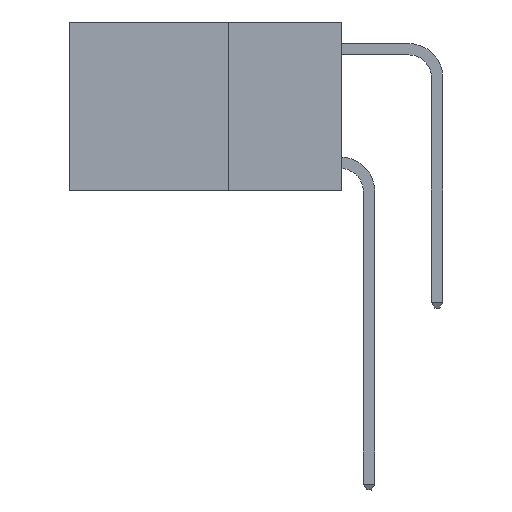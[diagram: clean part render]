
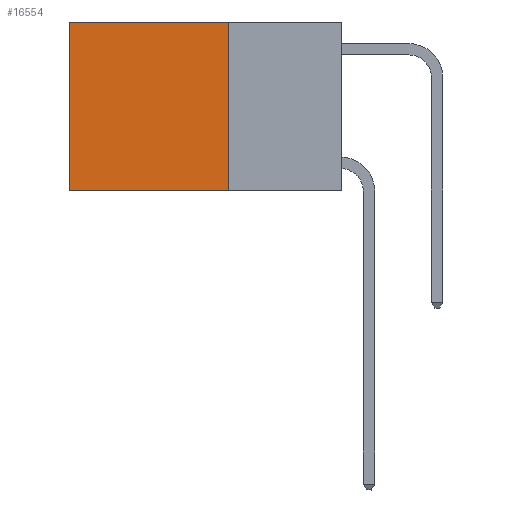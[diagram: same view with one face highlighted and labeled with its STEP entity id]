
A CAD part, left-side view. The second image highlights one B-rep face of the part: STEP entity #16554.
In plain terms, the highlighted planar face has unit normal (-1, 0, 0).
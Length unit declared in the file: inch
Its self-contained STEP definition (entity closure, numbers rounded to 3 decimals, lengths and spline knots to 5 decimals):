
#1660 = DIRECTION ( 'NONE',  ( 0., 1., 0. ) ) ;
#2607 = VECTOR ( 'NONE', #20338, 39.37008 ) ;
#3038 = VERTEX_POINT ( 'NONE', #21489 ) ;
#4496 = EDGE_CURVE ( 'NONE', #20024, #8910, #19858, .T. ) ;
#4910 = LINE ( 'NONE', #21414, #20687 ) ;
#5083 = EDGE_CURVE ( 'NONE', #3038, #20024, #23173, .T. ) ;
#5588 = CARTESIAN_POINT ( 'NONE',  ( 0.2625, 0.25, 0. ) ) ;
#6505 = CARTESIAN_POINT ( 'NONE',  ( 0.2625, 0.25, 0. ) ) ;
#6609 = ORIENTED_EDGE ( 'NONE', *, *, #5083, .T. ) ;
#6705 = AXIS2_PLACEMENT_3D ( 'NONE', #19787, #7940, #21731 ) ;
#7940 = DIRECTION ( 'NONE',  ( 1., 0., 0. ) ) ;
#8168 = EDGE_CURVE ( 'NONE', #3038, #17429, #18433, .T. ) ;
#8910 = VERTEX_POINT ( 'NONE', #14740 ) ;
#9590 = FACE_OUTER_BOUND ( 'NONE', #24114, .T. ) ;
#11730 = ORIENTED_EDGE ( 'NONE', *, *, #4496, .T. ) ;
#11795 = PLANE ( 'NONE',  #6705 ) ;
#11918 = EDGE_CURVE ( 'NONE', #17429, #8910, #4910, .T. ) ;
#12066 = VECTOR ( 'NONE', #1660, 39.37008 ) ;
#14740 = CARTESIAN_POINT ( 'NONE',  ( 0.2625, 0.6, -0.37 ) ) ;
#16554 = ADVANCED_FACE ( 'NONE', ( #9590 ), #11795, .F. ) ;
#16924 = ORIENTED_EDGE ( 'NONE', *, *, #8168, .F. ) ;
#17429 = VERTEX_POINT ( 'NONE', #22091 ) ;
#17833 = CARTESIAN_POINT ( 'NONE',  ( 0.2625, 0.6, 0. ) ) ;
#18433 = LINE ( 'NONE', #6505, #2607 ) ;
#19787 = CARTESIAN_POINT ( 'NONE',  ( 0.2625, 0.25, 0. ) ) ;
#19808 = DIRECTION ( 'NONE',  ( 0., 0., -1. ) ) ;
#19858 = LINE ( 'NONE', #17833, #24421 ) ;
#20024 = VERTEX_POINT ( 'NONE', #21630 ) ;
#20339 = ORIENTED_EDGE ( 'NONE', *, *, #11918, .F. ) ;
#20338 = DIRECTION ( 'NONE',  ( 0., 0., -1. ) ) ;
#20687 = VECTOR ( 'NONE', #23378, 39.37008 ) ;
#21414 = CARTESIAN_POINT ( 'NONE',  ( 0.2625, 0.25, -0.37 ) ) ;
#21489 = CARTESIAN_POINT ( 'NONE',  ( 0.2625, 0.25, 0. ) ) ;
#21630 = CARTESIAN_POINT ( 'NONE',  ( 0.2625, 0.6, 0. ) ) ;
#21731 = DIRECTION ( 'NONE',  ( 0., 0., -1. ) ) ;
#22091 = CARTESIAN_POINT ( 'NONE',  ( 0.2625, 0.25, -0.37 ) ) ;
#23173 = LINE ( 'NONE', #5588, #12066 ) ;
#23378 = DIRECTION ( 'NONE',  ( 0., 1., 0. ) ) ;
#24114 = EDGE_LOOP ( 'NONE', ( #11730, #20339, #16924, #6609 ) ) ;
#24421 = VECTOR ( 'NONE', #19808, 39.37008 ) ;
